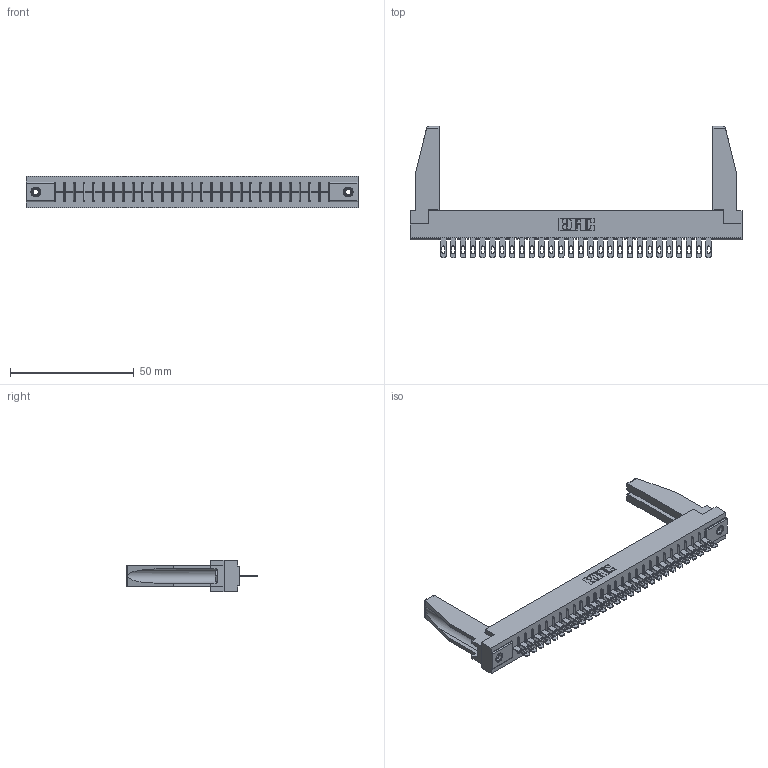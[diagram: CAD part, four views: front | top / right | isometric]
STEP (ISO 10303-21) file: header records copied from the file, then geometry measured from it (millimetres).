
FILE_DESCRIPTION (( 'STEP AP203' ), '1' );
FILE_NAME ('306-028-400-178.STEP', '2020-09-22T00:06:56', ( '' ), ( '' ), 'SwSTEP 2.0', 'SolidWorks 2020', '' );
FILE_SCHEMA (( 'CONFIG_CONTROL_DESIGN' ));
Length unit declared in the file: inch
Products named in the file (5): 306-028-400-178; 345-250-001_345-250-001-102; 306 Part_.156 Dia; 306-290-001_100; 307-220-078
Assembly tree (33 placements, depth 2):
  306-028-400-178
    306 Part_.156 Dia
    306-290-001_100  x28
    345-250-001_345-250-001-102  x2
    307-220-078  x2
Bounding box: 133.96 x 52.91 x 12.7 mm (x, y, z)
Volume: 18766.7 mm3; surface area: 19340.4 mm2
Topology: 33 solids, 33 shells, 2374 faces, 6666 edges, 4284 vertices
Faces by surface type: plane 1552, cylinder 694, sphere 112, cone 12, torus 4
Entity records: 30528 total; most frequent: CARTESIAN_POINT 5125, ORIENTED_EDGE 5038, DIRECTION 5007, EDGE_CURVE 2519, LINE 1963, VECTOR 1963, VERTEX_POINT 1598, AXIS2_PLACEMENT_3D 1522
